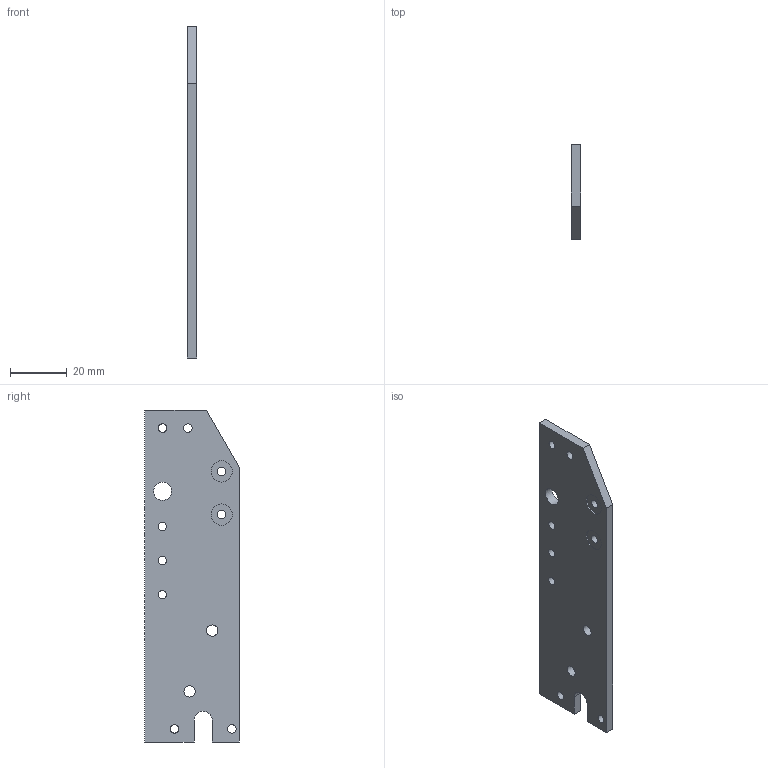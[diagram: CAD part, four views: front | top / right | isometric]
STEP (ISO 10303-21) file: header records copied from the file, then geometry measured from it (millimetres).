
FILE_DESCRIPTION (( 'STEP AP214' ), '1' );
FILE_NAME ('No_Safety_Reinforced_Side_Left.step', '2016-01-30T20:06:14', ( 'WarFairy' ), ( '' ), 'SwSTEP 2.0', 'SolidWorks 2015', '' );
FILE_SCHEMA (( 'AUTOMOTIVE_DESIGN' ));
Length unit declared in the file: millimetre
Products named in the file (1): No_Safety_Reinforced_Side_Left
Bounding box: 3.17 x 33.43 x 116.84 mm (x, y, z)
Volume: 11415.7 mm3; surface area: 8619.5 mm2
Topology: 1 solids, 1 shells, 27 faces, 71 edges, 48 vertices
Faces by surface type: cylinder 15, plane 12
Full cylindrical faces by diameter (mm): 3 x9, 3.97 x2, 6.35 x1, 7.5 x2
Entity records: 845 total; most frequent: DIRECTION 141, CARTESIAN_POINT 129, ORIENTED_EDGE 110, EDGE_LOOP 67, AXIS2_PLACEMENT_3D 58, EDGE_CURVE 55, VERTEX_POINT 46, FACE_OUTER_BOUND 41
